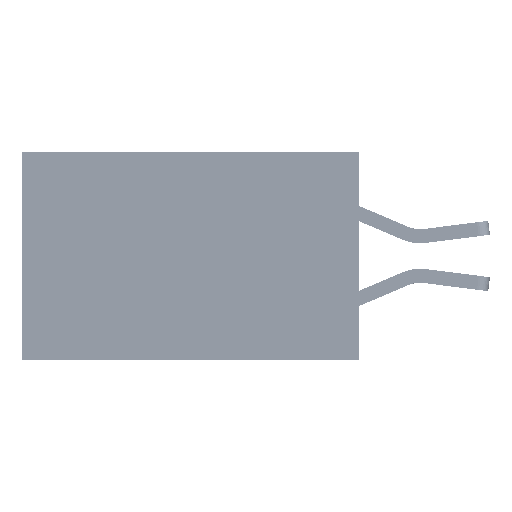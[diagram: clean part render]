
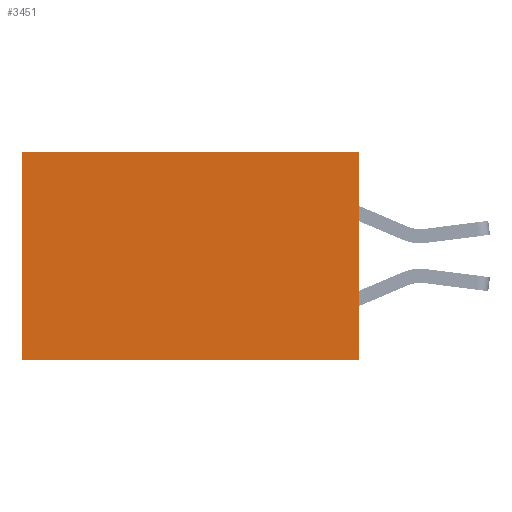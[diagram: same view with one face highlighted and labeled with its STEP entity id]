
A CAD part, left-side view. The second image highlights one B-rep face of the part: STEP entity #3451.
In plain terms, the highlighted planar face has unit normal (-1, 0, 0).
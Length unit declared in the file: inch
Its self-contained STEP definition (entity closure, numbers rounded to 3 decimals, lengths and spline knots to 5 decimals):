
#538 = AXIS2_PLACEMENT_3D ( 'NONE', #6124, #36324, #29831 ) ;
#3414 = CARTESIAN_POINT ( 'NONE',  ( 0.2875, 0.6, -0.37 ) ) ;
#3451 = ADVANCED_FACE ( 'NONE', ( #19340 ), #6400, .F. ) ;
#5398 = EDGE_LOOP ( 'NONE', ( #26529, #36964, #15722, #9370 ) ) ;
#6124 = CARTESIAN_POINT ( 'NONE',  ( 0.2875, 0., 0. ) ) ;
#6400 = PLANE ( 'NONE',  #538 ) ;
#6704 = CARTESIAN_POINT ( 'NONE',  ( 0.2875, 0., 0. ) ) ;
#8009 = LINE ( 'NONE', #14276, #28425 ) ;
#9370 = ORIENTED_EDGE ( 'NONE', *, *, #12307, .T. ) ;
#12307 = EDGE_CURVE ( 'NONE', #20361, #40288, #36238, .T. ) ;
#13285 = LINE ( 'NONE', #15297, #41591 ) ;
#14005 = CARTESIAN_POINT ( 'NONE',  ( 0.2875, 0., -0.37 ) ) ;
#14276 = CARTESIAN_POINT ( 'NONE',  ( 0.2875, 0.6, 0. ) ) ;
#14518 = CARTESIAN_POINT ( 'NONE',  ( 0.2875, 0., 0. ) ) ;
#15297 = CARTESIAN_POINT ( 'NONE',  ( 0.2875, 0., 0. ) ) ;
#15462 = CARTESIAN_POINT ( 'NONE',  ( 0.2875, 0.6, 0. ) ) ;
#15722 = ORIENTED_EDGE ( 'NONE', *, *, #27120, .F. ) ;
#17348 = VECTOR ( 'NONE', #33112, 39.37008 ) ;
#19340 = FACE_OUTER_BOUND ( 'NONE', #5398, .T. ) ;
#19745 = LINE ( 'NONE', #34449, #33316 ) ;
#20361 = VERTEX_POINT ( 'NONE', #14518 ) ;
#21022 = DIRECTION ( 'NONE',  ( 0., 0., -1. ) ) ;
#21482 = EDGE_CURVE ( 'NONE', #41302, #30905, #19745, .T. ) ;
#22179 = DIRECTION ( 'NONE',  ( 0., 0., -1. ) ) ;
#22591 = EDGE_CURVE ( 'NONE', #40288, #30905, #8009, .T. ) ;
#26529 = ORIENTED_EDGE ( 'NONE', *, *, #22591, .T. ) ;
#27120 = EDGE_CURVE ( 'NONE', #20361, #41302, #13285, .T. ) ;
#28425 = VECTOR ( 'NONE', #21022, 39.37008 ) ;
#29831 = DIRECTION ( 'NONE',  ( 0., 0., -1. ) ) ;
#30905 = VERTEX_POINT ( 'NONE', #3414 ) ;
#33112 = DIRECTION ( 'NONE',  ( 0., 1., 0. ) ) ;
#33316 = VECTOR ( 'NONE', #41182, 39.37008 ) ;
#34449 = CARTESIAN_POINT ( 'NONE',  ( 0.2875, 0., -0.37 ) ) ;
#36238 = LINE ( 'NONE', #6704, #17348 ) ;
#36324 = DIRECTION ( 'NONE',  ( 1., 0., 0. ) ) ;
#36964 = ORIENTED_EDGE ( 'NONE', *, *, #21482, .F. ) ;
#40288 = VERTEX_POINT ( 'NONE', #15462 ) ;
#41182 = DIRECTION ( 'NONE',  ( 0., 1., 0. ) ) ;
#41302 = VERTEX_POINT ( 'NONE', #14005 ) ;
#41591 = VECTOR ( 'NONE', #22179, 39.37008 ) ;
